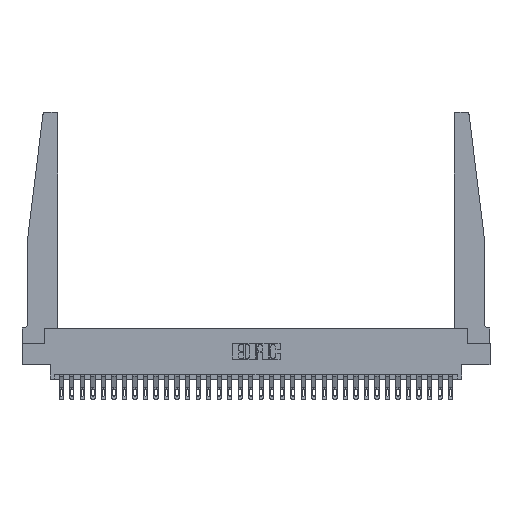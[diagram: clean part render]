
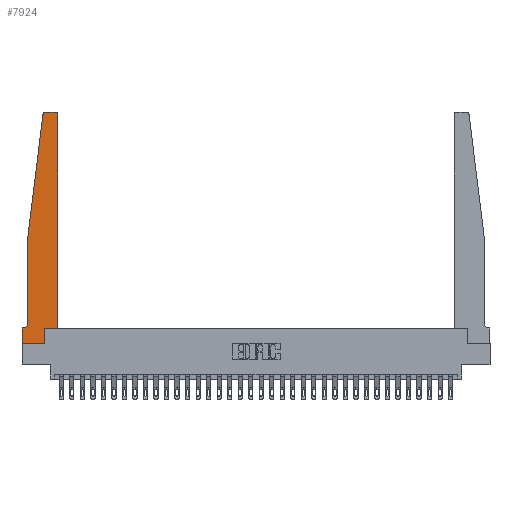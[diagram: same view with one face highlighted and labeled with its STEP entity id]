
A CAD part, top view. The second image highlights one B-rep face of the part: STEP entity #7924.
In plain terms, the highlighted planar face has unit normal (0, 0, 1).
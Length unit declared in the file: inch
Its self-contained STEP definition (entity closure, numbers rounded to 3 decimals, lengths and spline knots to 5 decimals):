
#288 = EDGE_CURVE ( 'NONE', #25614, #16355, #19348, .T. ) ;
#373 = CARTESIAN_POINT ( 'NONE',  ( 0.425, 0.18, 0.37 ) ) ;
#969 = ORIENTED_EDGE ( 'NONE', *, *, #29161, .T. ) ;
#1055 = EDGE_CURVE ( 'NONE', #28936, #1957, #29113, .T. ) ;
#1174 = ORIENTED_EDGE ( 'NONE', *, *, #3512, .T. ) ;
#1418 = AXIS2_PLACEMENT_3D ( 'NONE', #20889, #11143, #30287 ) ;
#1621 = VERTEX_POINT ( 'NONE', #15561 ) ;
#1858 = ORIENTED_EDGE ( 'NONE', *, *, #4571, .T. ) ;
#1957 = VERTEX_POINT ( 'NONE', #5320 ) ;
#1972 = DIRECTION ( 'NONE',  ( 0., 0., 1. ) ) ;
#2174 = LINE ( 'NONE', #26224, #12122 ) ;
#2442 = LINE ( 'NONE', #14530, #9080 ) ;
#3091 = CARTESIAN_POINT ( 'NONE',  ( 0.24675, 2.72367, 0.37 ) ) ;
#3478 = CARTESIAN_POINT ( 'NONE',  ( 0.015, 0.2375, 0.37 ) ) ;
#3512 = EDGE_CURVE ( 'NONE', #28069, #1621, #10708, .T. ) ;
#4036 = ORIENTED_EDGE ( 'NONE', *, *, #9640, .T. ) ;
#4158 = VERTEX_POINT ( 'NONE', #7333 ) ;
#4571 = EDGE_CURVE ( 'NONE', #1957, #4158, #13930, .T. ) ;
#4924 = ORIENTED_EDGE ( 'NONE', *, *, #288, .T. ) ;
#4984 = DIRECTION ( 'NONE',  ( -1., 0., 0. ) ) ;
#5044 = ORIENTED_EDGE ( 'NONE', *, *, #23188, .T. ) ;
#5154 = DIRECTION ( 'NONE',  ( 0., 0., 1. ) ) ;
#5279 = DIRECTION ( 'NONE',  ( 1., 0., 0. ) ) ;
#5320 = CARTESIAN_POINT ( 'NONE',  ( 0.425, 2.72, 0.37 ) ) ;
#5681 = VERTEX_POINT ( 'NONE', #3091 ) ;
#6131 = CARTESIAN_POINT ( 'NONE',  ( 0., 0., 0.37 ) ) ;
#6333 = CARTESIAN_POINT ( 'NONE',  ( 0.065, 1.25, 0.37 ) ) ;
#6762 = CARTESIAN_POINT ( 'NONE',  ( 0.27653, 2.75, 0.37 ) ) ;
#6829 = CARTESIAN_POINT ( 'NONE',  ( 0.2605, 0.18, 0.37 ) ) ;
#7333 = CARTESIAN_POINT ( 'NONE',  ( 0.395, 2.75, 0.37 ) ) ;
#7924 = ADVANCED_FACE ( 'NONE', ( #24039 ), #16791, .T. ) ;
#8691 = CARTESIAN_POINT ( 'NONE',  ( 0.2605, 0., 0.37 ) ) ;
#9080 = VECTOR ( 'NONE', #14375, 39.37008 ) ;
#9304 = DIRECTION ( 'NONE',  ( 1., 0., 0. ) ) ;
#9640 = EDGE_CURVE ( 'NONE', #27609, #28936, #17534, .T. ) ;
#10473 = CARTESIAN_POINT ( 'NONE',  ( 0.425, 0.18, 0.37 ) ) ;
#10708 = CIRCLE ( 'NONE', #21258, 0.05 ) ;
#10853 = CARTESIAN_POINT ( 'NONE',  ( 0., 0., 0.37 ) ) ;
#11143 = DIRECTION ( 'NONE',  ( 0., 0., 1. ) ) ;
#11498 = VECTOR ( 'NONE', #26315, 39.37008 ) ;
#11814 = VERTEX_POINT ( 'NONE', #23723 ) ;
#11862 = CARTESIAN_POINT ( 'NONE',  ( 0.395, 2.72, 0.37 ) ) ;
#12122 = VECTOR ( 'NONE', #14112, 39.37008 ) ;
#12287 = EDGE_CURVE ( 'NONE', #16355, #27609, #22917, .T. ) ;
#12452 = ORIENTED_EDGE ( 'NONE', *, *, #20314, .T. ) ;
#13529 = EDGE_CURVE ( 'NONE', #11814, #25614, #16614, .T. ) ;
#13930 = CIRCLE ( 'NONE', #28483, 0.03 ) ;
#14112 = DIRECTION ( 'NONE',  ( -1., 0., 0. ) ) ;
#14375 = DIRECTION ( 'NONE',  ( 0., -1., 0. ) ) ;
#14530 = CARTESIAN_POINT ( 'NONE',  ( 0.065, 1.25, 0.37 ) ) ;
#14801 = VECTOR ( 'NONE', #4984, 39.37008 ) ;
#14960 = CIRCLE ( 'NONE', #1418, 0.03 ) ;
#15561 = CARTESIAN_POINT ( 'NONE',  ( 0.015, 0.1875, 0.37 ) ) ;
#16355 = VERTEX_POINT ( 'NONE', #8691 ) ;
#16614 = LINE ( 'NONE', #10853, #22872 ) ;
#16630 = ORIENTED_EDGE ( 'NONE', *, *, #1055, .T. ) ;
#16725 = DIRECTION ( 'NONE',  ( 1., 0., 0. ) ) ;
#16791 = PLANE ( 'NONE',  #29285 ) ;
#16844 = DIRECTION ( 'NONE',  ( -0.122, -0.992, 0. ) ) ;
#17354 = VECTOR ( 'NONE', #9304, 39.37008 ) ;
#17534 = LINE ( 'NONE', #10473, #21166 ) ;
#18670 = CARTESIAN_POINT ( 'NONE',  ( 0.25, 2.75, 0.37 ) ) ;
#18691 = EDGE_CURVE ( 'NONE', #22017, #5681, #14960, .T. ) ;
#18782 = ORIENTED_EDGE ( 'NONE', *, *, #13529, .T. ) ;
#19348 = LINE ( 'NONE', #28926, #17354 ) ;
#19817 = DIRECTION ( 'NONE',  ( -1., 0., 0. ) ) ;
#20071 = VERTEX_POINT ( 'NONE', #6333 ) ;
#20314 = EDGE_CURVE ( 'NONE', #5681, #20071, #22349, .T. ) ;
#20889 = CARTESIAN_POINT ( 'NONE',  ( 0.27653, 2.72, 0.37 ) ) ;
#21166 = VECTOR ( 'NONE', #5279, 39.37008 ) ;
#21258 = AXIS2_PLACEMENT_3D ( 'NONE', #3478, #29543, #19817 ) ;
#21378 = DIRECTION ( 'NONE',  ( 1., 0., 0. ) ) ;
#21827 = VECTOR ( 'NONE', #25418, 39.37008 ) ;
#22017 = VERTEX_POINT ( 'NONE', #6762 ) ;
#22349 = LINE ( 'NONE', #24092, #25576 ) ;
#22384 = EDGE_CURVE ( 'NONE', #1621, #11814, #2174, .T. ) ;
#22872 = VECTOR ( 'NONE', #28561, 39.37008 ) ;
#22917 = LINE ( 'NONE', #27771, #21827 ) ;
#23188 = EDGE_CURVE ( 'NONE', #20071, #28069, #2442, .T. ) ;
#23453 = CARTESIAN_POINT ( 'NONE',  ( 0.065, 0.2375, 0.37 ) ) ;
#23723 = CARTESIAN_POINT ( 'NONE',  ( 0., 0.1875, 0.37 ) ) ;
#24039 = FACE_OUTER_BOUND ( 'NONE', #25628, .T. ) ;
#24092 = CARTESIAN_POINT ( 'NONE',  ( 0.065, 1.25, 0.37 ) ) ;
#25037 = ORIENTED_EDGE ( 'NONE', *, *, #18691, .T. ) ;
#25418 = DIRECTION ( 'NONE',  ( 0., 1., 0. ) ) ;
#25576 = VECTOR ( 'NONE', #16844, 39.37008 ) ;
#25614 = VERTEX_POINT ( 'NONE', #6131 ) ;
#25628 = EDGE_LOOP ( 'NONE', ( #969, #25037, #12452, #5044, #1174, #27188, #18782, #4924, #26246, #4036, #16630, #1858 ) ) ;
#25890 = LINE ( 'NONE', #18670, #14801 ) ;
#26224 = CARTESIAN_POINT ( 'NONE',  ( 0.065, 0.1875, 0.37 ) ) ;
#26246 = ORIENTED_EDGE ( 'NONE', *, *, #12287, .T. ) ;
#26315 = DIRECTION ( 'NONE',  ( 0., 1., 0. ) ) ;
#26689 = CARTESIAN_POINT ( 'NONE',  ( 0., 0.1875, 0.37 ) ) ;
#27188 = ORIENTED_EDGE ( 'NONE', *, *, #22384, .T. ) ;
#27609 = VERTEX_POINT ( 'NONE', #6829 ) ;
#27771 = CARTESIAN_POINT ( 'NONE',  ( 0.2605, 0.18, 0.37 ) ) ;
#28069 = VERTEX_POINT ( 'NONE', #23453 ) ;
#28483 = AXIS2_PLACEMENT_3D ( 'NONE', #11862, #1972, #16725 ) ;
#28561 = DIRECTION ( 'NONE',  ( 0., -1., 0. ) ) ;
#28926 = CARTESIAN_POINT ( 'NONE',  ( 0., 0., 0.37 ) ) ;
#28936 = VERTEX_POINT ( 'NONE', #30429 ) ;
#29113 = LINE ( 'NONE', #373, #11498 ) ;
#29161 = EDGE_CURVE ( 'NONE', #4158, #22017, #25890, .T. ) ;
#29285 = AXIS2_PLACEMENT_3D ( 'NONE', #26689, #5154, #21378 ) ;
#29543 = DIRECTION ( 'NONE',  ( 0., 0., -1. ) ) ;
#30287 = DIRECTION ( 'NONE',  ( 1., 0., 0. ) ) ;
#30429 = CARTESIAN_POINT ( 'NONE',  ( 0.425, 0.18, 0.37 ) ) ;
